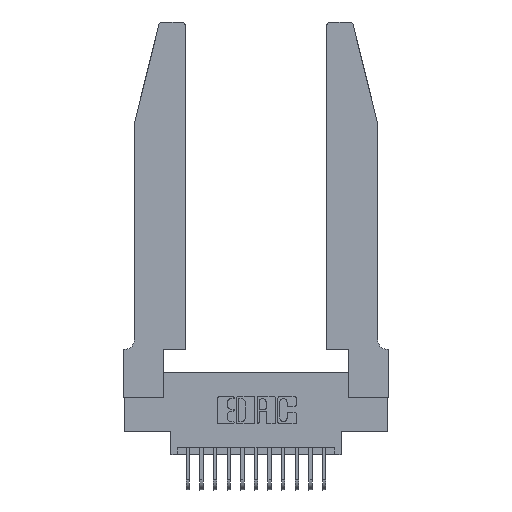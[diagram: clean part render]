
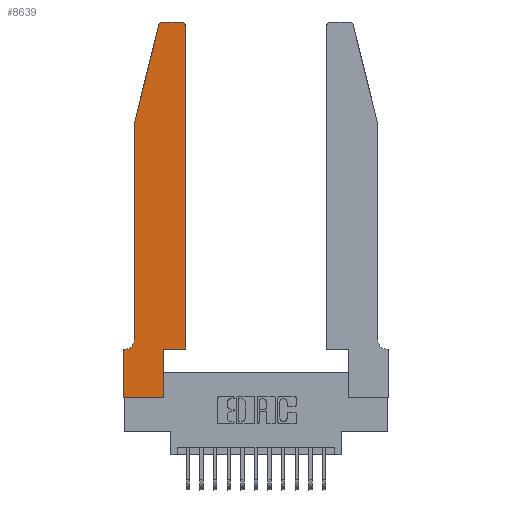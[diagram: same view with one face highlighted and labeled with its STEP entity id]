
A CAD part, top view. The second image highlights one B-rep face of the part: STEP entity #8639.
In plain terms, the highlighted planar face has unit normal (0, 0, 1).
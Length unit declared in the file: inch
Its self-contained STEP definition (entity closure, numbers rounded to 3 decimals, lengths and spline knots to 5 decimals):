
#63 = VECTOR ( 'NONE', #14887, 39.37008 ) ;
#246 = EDGE_CURVE ( 'NONE', #18138, #6838, #12004, .T. ) ;
#455 = ORIENTED_EDGE ( 'NONE', *, *, #12511, .T. ) ;
#458 = DIRECTION ( 'NONE',  ( -1., 0., 0. ) ) ;
#577 = VECTOR ( 'NONE', #18249, 39.37008 ) ;
#739 = EDGE_CURVE ( 'NONE', #17976, #838, #15930, .T. ) ;
#803 = CARTESIAN_POINT ( 'NONE',  ( 0.4205, 2.75, 0.37 ) ) ;
#838 = VERTEX_POINT ( 'NONE', #4415 ) ;
#956 = ORIENTED_EDGE ( 'NONE', *, *, #2744, .T. ) ;
#989 = CARTESIAN_POINT ( 'NONE',  ( 0.25487, 2.72718, 0.37 ) ) ;
#1373 = DIRECTION ( 'NONE',  ( 1., 0., 0. ) ) ;
#1904 = AXIS2_PLACEMENT_3D ( 'NONE', #19295, #10367, #1373 ) ;
#1954 = VECTOR ( 'NONE', #5611, 39.37008 ) ;
#2267 = CARTESIAN_POINT ( 'NONE',  ( 0.4505, 0.35, 0.37 ) ) ;
#2301 = DIRECTION ( 'NONE',  ( -1., 0., 0. ) ) ;
#2744 = EDGE_CURVE ( 'NONE', #15399, #8874, #14726, .T. ) ;
#2955 = CARTESIAN_POINT ( 'NONE',  ( 0.284, 2.72, 0.37 ) ) ;
#3062 = CARTESIAN_POINT ( 'NONE',  ( 0.0755, 0.42, 0.37 ) ) ;
#3213 = VECTOR ( 'NONE', #7962, 39.37008 ) ;
#3265 = PLANE ( 'NONE',  #14690 ) ;
#3404 = CARTESIAN_POINT ( 'NONE',  ( 0.0055, 0.35, 0.37 ) ) ;
#3676 = CARTESIAN_POINT ( 'NONE',  ( 0.2865, 0.35, 0.37 ) ) ;
#3759 = CARTESIAN_POINT ( 'NONE',  ( 0.4505, 2.72, 0.37 ) ) ;
#3942 = EDGE_CURVE ( 'NONE', #13620, #17588, #5012, .T. ) ;
#4125 = ORIENTED_EDGE ( 'NONE', *, *, #17048, .T. ) ;
#4323 = EDGE_LOOP ( 'NONE', ( #956, #8703, #455, #7062, #17355, #17852, #4125, #15104, #9929, #13464, #10757, #4361 ) ) ;
#4361 = ORIENTED_EDGE ( 'NONE', *, *, #8994, .T. ) ;
#4415 = CARTESIAN_POINT ( 'NONE',  ( 0.2865, 0., 0.37 ) ) ;
#4452 = CIRCLE ( 'NONE', #18972, 0.03 ) ;
#4468 = DIRECTION ( 'NONE',  ( 1., 0., 0. ) ) ;
#4480 = DIRECTION ( 'NONE',  ( 0., 1., 0. ) ) ;
#4607 = VECTOR ( 'NONE', #4956, 39.37008 ) ;
#4779 = DIRECTION ( 'NONE',  ( 1., 0., 0. ) ) ;
#4813 = VERTEX_POINT ( 'NONE', #3759 ) ;
#4851 = EDGE_CURVE ( 'NONE', #838, #18138, #13881, .T. ) ;
#4956 = DIRECTION ( 'NONE',  ( 0., -1., 0. ) ) ;
#5012 = LINE ( 'NONE', #6265, #577 ) ;
#5258 = VECTOR ( 'NONE', #4480, 39.37008 ) ;
#5552 = CARTESIAN_POINT ( 'NONE',  ( 0.284, 2.75, 0.37 ) ) ;
#5611 = DIRECTION ( 'NONE',  ( -0.239, -0.971, 0. ) ) ;
#6265 = CARTESIAN_POINT ( 'NONE',  ( 0.0755, 0.35, 0.37 ) ) ;
#6838 = VERTEX_POINT ( 'NONE', #2267 ) ;
#7062 = ORIENTED_EDGE ( 'NONE', *, *, #9254, .T. ) ;
#7219 = LINE ( 'NONE', #16906, #3213 ) ;
#7244 = VECTOR ( 'NONE', #2301, 39.37008 ) ;
#7781 = VERTEX_POINT ( 'NONE', #14819 ) ;
#7962 = DIRECTION ( 'NONE',  ( 0., -1., 0. ) ) ;
#8630 = DIRECTION ( 'NONE',  ( 1., 0., 0. ) ) ;
#8639 = ADVANCED_FACE ( 'NONE', ( #10511 ), #3265, .T. ) ;
#8703 = ORIENTED_EDGE ( 'NONE', *, *, #17954, .T. ) ;
#8874 = VERTEX_POINT ( 'NONE', #5552 ) ;
#8994 = EDGE_CURVE ( 'NONE', #4813, #15399, #16806, .T. ) ;
#9030 = CARTESIAN_POINT ( 'NONE',  ( 0., 0., 0.37 ) ) ;
#9048 = AXIS2_PLACEMENT_3D ( 'NONE', #18371, #9442, #458 ) ;
#9095 = VERTEX_POINT ( 'NONE', #3062 ) ;
#9254 = EDGE_CURVE ( 'NONE', #7781, #9095, #12127, .T. ) ;
#9442 = DIRECTION ( 'NONE',  ( 0., 0., -1. ) ) ;
#9454 = CARTESIAN_POINT ( 'NONE',  ( 0., 0.35, 0.37 ) ) ;
#9807 = DIRECTION ( 'NONE',  ( 0., 1., 0. ) ) ;
#9929 = ORIENTED_EDGE ( 'NONE', *, *, #4851, .T. ) ;
#9950 = LINE ( 'NONE', #14578, #1954 ) ;
#10367 = DIRECTION ( 'NONE',  ( 0., 0., 1. ) ) ;
#10402 = VECTOR ( 'NONE', #9807, 39.37008 ) ;
#10511 = FACE_OUTER_BOUND ( 'NONE', #4323, .T. ) ;
#10757 = ORIENTED_EDGE ( 'NONE', *, *, #11884, .T. ) ;
#11460 = EDGE_CURVE ( 'NONE', #9095, #13620, #14876, .T. ) ;
#11884 = EDGE_CURVE ( 'NONE', #6838, #4813, #12303, .T. ) ;
#11979 = VECTOR ( 'NONE', #8630, 39.37008 ) ;
#12004 = LINE ( 'NONE', #16159, #63 ) ;
#12127 = LINE ( 'NONE', #13923, #4607 ) ;
#12303 = LINE ( 'NONE', #13450, #5258 ) ;
#12511 = EDGE_CURVE ( 'NONE', #13894, #7781, #9950, .T. ) ;
#13443 = DIRECTION ( 'NONE',  ( 0., 0., 1. ) ) ;
#13450 = CARTESIAN_POINT ( 'NONE',  ( 0.4505, 0.35, 0.37 ) ) ;
#13464 = ORIENTED_EDGE ( 'NONE', *, *, #246, .T. ) ;
#13620 = VERTEX_POINT ( 'NONE', #3404 ) ;
#13747 = DIRECTION ( 'NONE',  ( 0., 0., 1. ) ) ;
#13881 = LINE ( 'NONE', #18737, #10402 ) ;
#13894 = VERTEX_POINT ( 'NONE', #989 ) ;
#13923 = CARTESIAN_POINT ( 'NONE',  ( 0.0755, 2., 0.37 ) ) ;
#14578 = CARTESIAN_POINT ( 'NONE',  ( 0.0755, 2., 0.37 ) ) ;
#14690 = AXIS2_PLACEMENT_3D ( 'NONE', #18199, #13747, #4779 ) ;
#14726 = LINE ( 'NONE', #17446, #7244 ) ;
#14819 = CARTESIAN_POINT ( 'NONE',  ( 0.0755, 2., 0.37 ) ) ;
#14876 = CIRCLE ( 'NONE', #9048, 0.07 ) ;
#14887 = DIRECTION ( 'NONE',  ( 1., 0., 0. ) ) ;
#15104 = ORIENTED_EDGE ( 'NONE', *, *, #739, .T. ) ;
#15399 = VERTEX_POINT ( 'NONE', #803 ) ;
#15930 = LINE ( 'NONE', #17070, #11979 ) ;
#16159 = CARTESIAN_POINT ( 'NONE',  ( 0.4505, 0.35, 0.37 ) ) ;
#16806 = CIRCLE ( 'NONE', #1904, 0.03 ) ;
#16906 = CARTESIAN_POINT ( 'NONE',  ( 0., 0., 0.37 ) ) ;
#17048 = EDGE_CURVE ( 'NONE', #17588, #17976, #7219, .T. ) ;
#17070 = CARTESIAN_POINT ( 'NONE',  ( 0., 0., 0.37 ) ) ;
#17355 = ORIENTED_EDGE ( 'NONE', *, *, #11460, .T. ) ;
#17446 = CARTESIAN_POINT ( 'NONE',  ( 0.2605, 2.75, 0.37 ) ) ;
#17588 = VERTEX_POINT ( 'NONE', #9454 ) ;
#17852 = ORIENTED_EDGE ( 'NONE', *, *, #3942, .T. ) ;
#17954 = EDGE_CURVE ( 'NONE', #8874, #13894, #4452, .T. ) ;
#17976 = VERTEX_POINT ( 'NONE', #9030 ) ;
#18138 = VERTEX_POINT ( 'NONE', #3676 ) ;
#18199 = CARTESIAN_POINT ( 'NONE',  ( 0., 0.35, 0.37 ) ) ;
#18249 = DIRECTION ( 'NONE',  ( -1., 0., 0. ) ) ;
#18371 = CARTESIAN_POINT ( 'NONE',  ( 0.0055, 0.42, 0.37 ) ) ;
#18737 = CARTESIAN_POINT ( 'NONE',  ( 0.2865, 0.35, 0.37 ) ) ;
#18972 = AXIS2_PLACEMENT_3D ( 'NONE', #2955, #13443, #4468 ) ;
#19295 = CARTESIAN_POINT ( 'NONE',  ( 0.4205, 2.72, 0.37 ) ) ;
